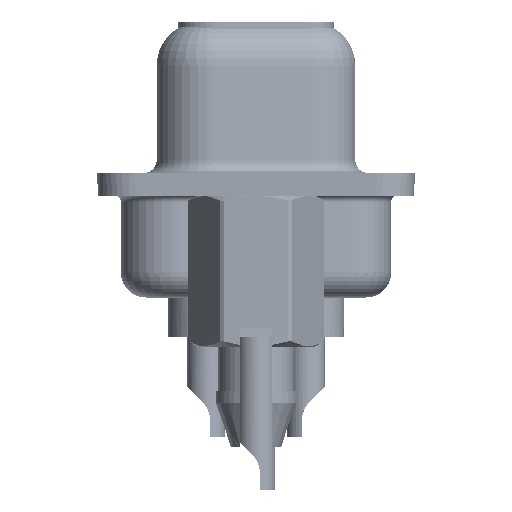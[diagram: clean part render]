
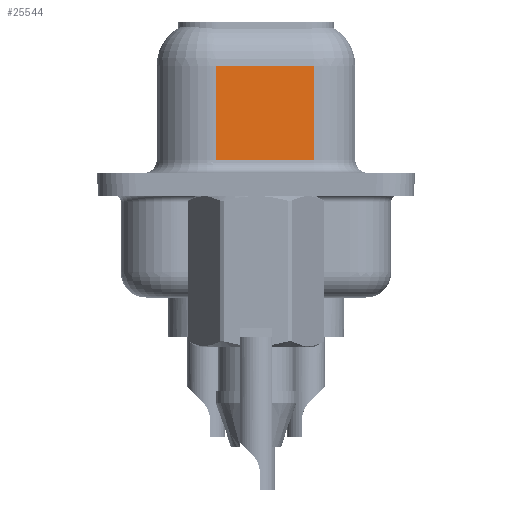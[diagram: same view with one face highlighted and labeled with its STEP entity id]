
A CAD part, left-side view. The second image highlights one B-rep face of the part: STEP entity #25544.
In plain terms, the highlighted planar face has unit normal (-0.985, -0.174, 0).
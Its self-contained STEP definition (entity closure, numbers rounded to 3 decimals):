
#1323 = DIRECTION ( 'NONE',  ( 0., 0., -1. ) ) ;
#2081 = PLANE ( 'NONE',  #27850 ) ;
#2725 = FACE_OUTER_BOUND ( 'NONE', #14834, .T. ) ;
#7998 = DIRECTION ( 'NONE',  ( 0., 0., -1. ) ) ;
#9536 = VERTEX_POINT ( 'NONE', #28470 ) ;
#11369 = LINE ( 'NONE', #25088, #29486 ) ;
#13858 = DIRECTION ( 'NONE',  ( 0.174, -0.985, 0. ) ) ;
#14612 = VERTEX_POINT ( 'NONE', #29359 ) ;
#14834 = EDGE_LOOP ( 'NONE', ( #19646, #20009, #37457, #29759 ) ) ;
#15106 = VECTOR ( 'NONE', #13858, 1000. ) ;
#17223 = LINE ( 'NONE', #28469, #15106 ) ;
#17538 = EDGE_CURVE ( 'NONE', #14612, #31955, #17223, .T. ) ;
#18383 = CARTESIAN_POINT ( 'NONE',  ( 4.38, 1.603, 6.45 ) ) ;
#18604 = LINE ( 'NONE', #18383, #43198 ) ;
#19646 = ORIENTED_EDGE ( 'NONE', *, *, #43468, .F. ) ;
#20009 = ORIENTED_EDGE ( 'NONE', *, *, #34165, .T. ) ;
#20476 = LINE ( 'NONE', #21134, #31320 ) ;
#21134 = CARTESIAN_POINT ( 'NONE',  ( 5.068, -2.297, 4.7 ) ) ;
#24856 = CARTESIAN_POINT ( 'NONE',  ( 5.068, -2.297, 0.95 ) ) ;
#25088 = CARTESIAN_POINT ( 'NONE',  ( 5.068, -2.297, 6.45 ) ) ;
#25544 = ADVANCED_FACE ( 'NONE', ( #2725 ), #2081, .F. ) ;
#27850 = AXIS2_PLACEMENT_3D ( 'NONE', #29051, #29926, #39382 ) ;
#28469 = CARTESIAN_POINT ( 'NONE',  ( 5.068, -2.297, 0.95 ) ) ;
#28470 = CARTESIAN_POINT ( 'NONE',  ( 4.38, 1.603, 4.7 ) ) ;
#29051 = CARTESIAN_POINT ( 'NONE',  ( 5.068, -2.297, 6.45 ) ) ;
#29359 = CARTESIAN_POINT ( 'NONE',  ( 4.38, 1.603, 0.95 ) ) ;
#29486 = VECTOR ( 'NONE', #7998, 1000. ) ;
#29759 = ORIENTED_EDGE ( 'NONE', *, *, #17538, .T. ) ;
#29926 = DIRECTION ( 'NONE',  ( 0.985, 0.174, 0. ) ) ;
#31320 = VECTOR ( 'NONE', #34222, 1000. ) ;
#31955 = VERTEX_POINT ( 'NONE', #24856 ) ;
#32139 = CARTESIAN_POINT ( 'NONE',  ( 5.068, -2.297, 4.7 ) ) ;
#34165 = EDGE_CURVE ( 'NONE', #42446, #9536, #20476, .T. ) ;
#34222 = DIRECTION ( 'NONE',  ( -0.174, 0.985, 0. ) ) ;
#37457 = ORIENTED_EDGE ( 'NONE', *, *, #44314, .T. ) ;
#39382 = DIRECTION ( 'NONE',  ( -0.174, 0.985, 0. ) ) ;
#42446 = VERTEX_POINT ( 'NONE', #32139 ) ;
#43198 = VECTOR ( 'NONE', #1323, 1000. ) ;
#43468 = EDGE_CURVE ( 'NONE', #42446, #31955, #11369, .T. ) ;
#44314 = EDGE_CURVE ( 'NONE', #9536, #14612, #18604, .T. ) ;
